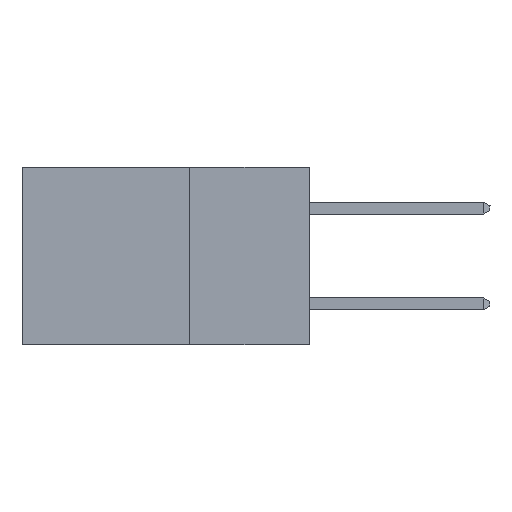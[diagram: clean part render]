
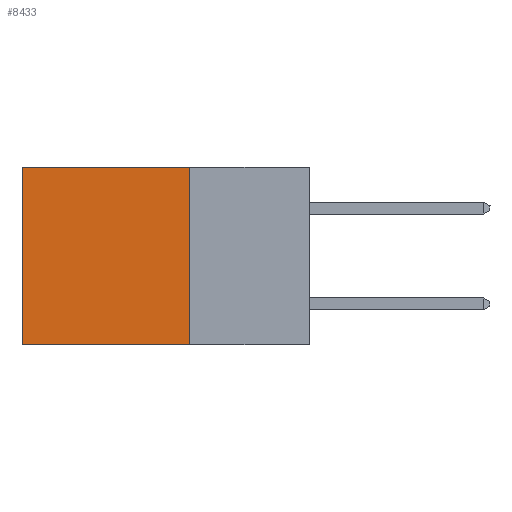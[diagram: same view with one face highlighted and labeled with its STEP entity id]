
A CAD part, left-side view. The second image highlights one B-rep face of the part: STEP entity #8433.
In plain terms, the highlighted planar face has unit normal (-1, 0, 0).
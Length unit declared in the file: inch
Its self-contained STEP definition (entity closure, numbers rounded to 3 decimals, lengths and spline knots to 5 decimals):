
#269 = EDGE_CURVE ( 'NONE', #11134, #11461, #16148, .T. ) ;
#429 = CARTESIAN_POINT ( 'NONE',  ( 0.2875, 0.25, -0.37 ) ) ;
#502 = LINE ( 'NONE', #6012, #8153 ) ;
#510 = DIRECTION ( 'NONE',  ( 1., 0., 0. ) ) ;
#698 = DIRECTION ( 'NONE',  ( 0., 0., -1. ) ) ;
#797 = CARTESIAN_POINT ( 'NONE',  ( 0.2875, 0.25, -0.37 ) ) ;
#1072 = CARTESIAN_POINT ( 'NONE',  ( 0.2875, 0.25, 0. ) ) ;
#1668 = VERTEX_POINT ( 'NONE', #3548 ) ;
#1910 = CARTESIAN_POINT ( 'NONE',  ( 0.2875, 0.25, 0. ) ) ;
#3434 = EDGE_CURVE ( 'NONE', #8304, #1668, #502, .T. ) ;
#3548 = CARTESIAN_POINT ( 'NONE',  ( 0.2875, 0.6, 0. ) ) ;
#4053 = EDGE_LOOP ( 'NONE', ( #14986, #11598, #16342, #11108 ) ) ;
#5244 = DIRECTION ( 'NONE',  ( 0., 0., -1. ) ) ;
#5826 = DIRECTION ( 'NONE',  ( 0., 1., 0. ) ) ;
#6012 = CARTESIAN_POINT ( 'NONE',  ( 0.2875, 0.25, 0. ) ) ;
#7322 = PLANE ( 'NONE',  #9540 ) ;
#7329 = CARTESIAN_POINT ( 'NONE',  ( 0.2875, 0.6, -0.37 ) ) ;
#7876 = CARTESIAN_POINT ( 'NONE',  ( 0.2875, 0.6, 0. ) ) ;
#8153 = VECTOR ( 'NONE', #5826, 39.37008 ) ;
#8304 = VERTEX_POINT ( 'NONE', #12191 ) ;
#8433 = ADVANCED_FACE ( 'NONE', ( #12449 ), #7322, .F. ) ;
#9464 = EDGE_CURVE ( 'NONE', #8304, #11134, #16799, .T. ) ;
#9540 = AXIS2_PLACEMENT_3D ( 'NONE', #1910, #510, #698 ) ;
#9869 = DIRECTION ( 'NONE',  ( 0., 1., 0. ) ) ;
#10388 = VECTOR ( 'NONE', #15747, 39.37008 ) ;
#11108 = ORIENTED_EDGE ( 'NONE', *, *, #3434, .T. ) ;
#11119 = VECTOR ( 'NONE', #5244, 39.37008 ) ;
#11134 = VERTEX_POINT ( 'NONE', #797 ) ;
#11461 = VERTEX_POINT ( 'NONE', #7329 ) ;
#11598 = ORIENTED_EDGE ( 'NONE', *, *, #269, .F. ) ;
#12163 = EDGE_CURVE ( 'NONE', #1668, #11461, #17127, .T. ) ;
#12191 = CARTESIAN_POINT ( 'NONE',  ( 0.2875, 0.25, 0. ) ) ;
#12316 = VECTOR ( 'NONE', #9869, 39.37008 ) ;
#12449 = FACE_OUTER_BOUND ( 'NONE', #4053, .T. ) ;
#14986 = ORIENTED_EDGE ( 'NONE', *, *, #12163, .T. ) ;
#15747 = DIRECTION ( 'NONE',  ( 0., 0., -1. ) ) ;
#16148 = LINE ( 'NONE', #429, #12316 ) ;
#16342 = ORIENTED_EDGE ( 'NONE', *, *, #9464, .F. ) ;
#16799 = LINE ( 'NONE', #1072, #10388 ) ;
#17127 = LINE ( 'NONE', #7876, #11119 ) ;
